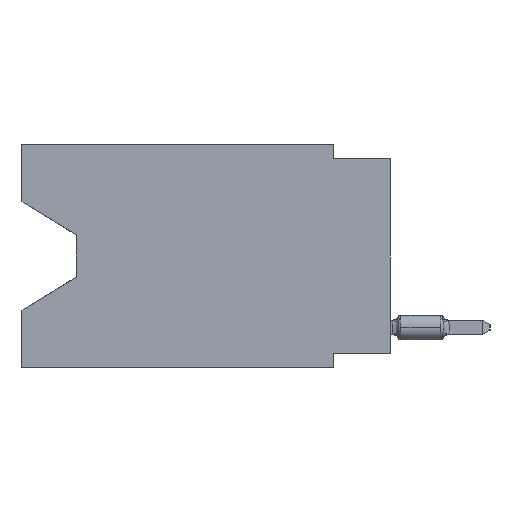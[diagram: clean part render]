
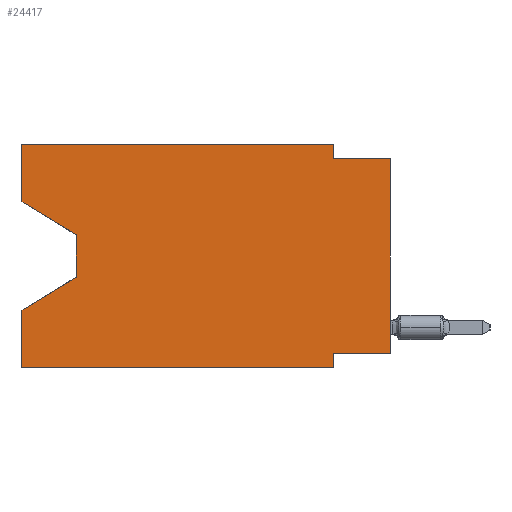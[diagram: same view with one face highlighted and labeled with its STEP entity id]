
A CAD part, left-side view. The second image highlights one B-rep face of the part: STEP entity #24417.
In plain terms, the highlighted planar face has unit normal (-1, 0, 0).
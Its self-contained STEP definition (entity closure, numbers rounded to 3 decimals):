
#320 = CARTESIAN_POINT ( 'NONE',  ( 0., 2.54, -9.906 ) ) ;
#419 = ORIENTED_EDGE ( 'NONE', *, *, #29567, .F. ) ;
#434 = VERTEX_POINT ( 'NONE', #31458 ) ;
#582 = CARTESIAN_POINT ( 'NONE',  ( 0., 16.383, -2.546 ) ) ;
#622 = LINE ( 'NONE', #24357, #13820 ) ;
#1254 = LINE ( 'NONE', #16887, #22067 ) ;
#1901 = ORIENTED_EDGE ( 'NONE', *, *, #32704, .F. ) ;
#2399 = DIRECTION ( 'NONE',  ( 0., 0., 1. ) ) ;
#2445 = ORIENTED_EDGE ( 'NONE', *, *, #22307, .F. ) ;
#2639 = VERTEX_POINT ( 'NONE', #28335 ) ;
#2742 = CARTESIAN_POINT ( 'NONE',  ( 0., 16.383, 0. ) ) ;
#2745 = ORIENTED_EDGE ( 'NONE', *, *, #31666, .T. ) ;
#2800 = VECTOR ( 'NONE', #32948, 1000. ) ;
#3052 = ORIENTED_EDGE ( 'NONE', *, *, #31285, .T. ) ;
#3186 = LINE ( 'NONE', #11596, #4100 ) ;
#3419 = EDGE_CURVE ( 'NONE', #2639, #34165, #1254, .T. ) ;
#3425 = EDGE_CURVE ( 'NONE', #27504, #32632, #14602, .T. ) ;
#4008 = ORIENTED_EDGE ( 'NONE', *, *, #20793, .F. ) ;
#4100 = VECTOR ( 'NONE', #17050, 1000. ) ;
#4119 = CARTESIAN_POINT ( 'NONE',  ( 0., 2.54, -9.271 ) ) ;
#5237 = VECTOR ( 'NONE', #19702, 1000. ) ;
#5678 = CARTESIAN_POINT ( 'NONE',  ( 0., 16.383, 0. ) ) ;
#5888 = VECTOR ( 'NONE', #28918, 1000. ) ;
#8313 = LINE ( 'NONE', #5678, #13576 ) ;
#8355 = CARTESIAN_POINT ( 'NONE',  ( 0., 16.383, -9.906 ) ) ;
#9902 = LINE ( 'NONE', #23429, #23069 ) ;
#10586 = ORIENTED_EDGE ( 'NONE', *, *, #19698, .F. ) ;
#10642 = CARTESIAN_POINT ( 'NONE',  ( 0., 2.54, 0. ) ) ;
#11029 = DIRECTION ( 'NONE',  ( 0., 0., -1. ) ) ;
#11428 = DIRECTION ( 'NONE',  ( 0., 0., 1. ) ) ;
#11596 = CARTESIAN_POINT ( 'NONE',  ( 0., 0., -0.635 ) ) ;
#12341 = CARTESIAN_POINT ( 'NONE',  ( 0., 16.383, -7.36 ) ) ;
#12742 = CARTESIAN_POINT ( 'NONE',  ( 0., 13.97, -5.893 ) ) ;
#12878 = DIRECTION ( 'NONE',  ( 0., 0., -1. ) ) ;
#13576 = VECTOR ( 'NONE', #27130, 1000. ) ;
#13820 = VECTOR ( 'NONE', #19258, 1000. ) ;
#13827 = VECTOR ( 'NONE', #11029, 1000. ) ;
#14162 = CARTESIAN_POINT ( 'NONE',  ( 0., 16.383, 0. ) ) ;
#14336 = LINE ( 'NONE', #21589, #2800 ) ;
#14414 = FACE_OUTER_BOUND ( 'NONE', #19501, .T. ) ;
#14585 = DIRECTION ( 'NONE',  ( 1., 0., 0. ) ) ;
#14602 = LINE ( 'NONE', #30751, #5237 ) ;
#16218 = VERTEX_POINT ( 'NONE', #21781 ) ;
#16665 = VERTEX_POINT ( 'NONE', #12341 ) ;
#16887 = CARTESIAN_POINT ( 'NONE',  ( 0., 0., 0. ) ) ;
#17050 = DIRECTION ( 'NONE',  ( 0., -1., 0. ) ) ;
#17220 = PLANE ( 'NONE',  #29820 ) ;
#17587 = DIRECTION ( 'NONE',  ( 0., -0.855, -0.519 ) ) ;
#17879 = VECTOR ( 'NONE', #27169, 1000. ) ;
#18353 = CARTESIAN_POINT ( 'NONE',  ( 0., 0., -0.635 ) ) ;
#19258 = DIRECTION ( 'NONE',  ( 0., -1., 0. ) ) ;
#19458 = VERTEX_POINT ( 'NONE', #28154 ) ;
#19501 = EDGE_LOOP ( 'NONE', ( #2745, #30561, #34324, #31745, #3052, #419, #1901, #31665, #10586, #2445, #21273, #4008 ) ) ;
#19682 = CARTESIAN_POINT ( 'NONE',  ( 0., 16.383, 0. ) ) ;
#19698 = EDGE_CURVE ( 'NONE', #26104, #34165, #3186, .T. ) ;
#19702 = DIRECTION ( 'NONE',  ( 0., -1., 0. ) ) ;
#20224 = LINE ( 'NONE', #23204, #25614 ) ;
#20793 = EDGE_CURVE ( 'NONE', #33190, #27504, #26462, .T. ) ;
#21034 = VERTEX_POINT ( 'NONE', #4119 ) ;
#21273 = ORIENTED_EDGE ( 'NONE', *, *, #3425, .F. ) ;
#21589 = CARTESIAN_POINT ( 'NONE',  ( 0., 13.97, -4.013 ) ) ;
#21781 = CARTESIAN_POINT ( 'NONE',  ( 0., 2.54, -9.906 ) ) ;
#22067 = VECTOR ( 'NONE', #11428, 1000. ) ;
#22307 = EDGE_CURVE ( 'NONE', #32632, #26104, #9902, .T. ) ;
#22469 = EDGE_CURVE ( 'NONE', #31222, #16665, #8313, .T. ) ;
#23069 = VECTOR ( 'NONE', #12878, 1000. ) ;
#23204 = CARTESIAN_POINT ( 'NONE',  ( 0., 16.383, -2.546 ) ) ;
#23429 = CARTESIAN_POINT ( 'NONE',  ( 0., 2.54, 0. ) ) ;
#23546 = VECTOR ( 'NONE', #2399, 1000. ) ;
#24357 = CARTESIAN_POINT ( 'NONE',  ( 0., 16.383, -9.906 ) ) ;
#24417 = ADVANCED_FACE ( 'NONE', ( #14414 ), #17220, .F. ) ;
#25614 = VECTOR ( 'NONE', #17587, 1000. ) ;
#26104 = VERTEX_POINT ( 'NONE', #28411 ) ;
#26462 = LINE ( 'NONE', #2742, #23546 ) ;
#26990 = LINE ( 'NONE', #29791, #17879 ) ;
#27130 = DIRECTION ( 'NONE',  ( 0., 0., 1. ) ) ;
#27169 = DIRECTION ( 'NONE',  ( 0., 1., 0. ) ) ;
#27377 = LINE ( 'NONE', #320, #13827 ) ;
#27504 = VERTEX_POINT ( 'NONE', #14162 ) ;
#28145 = EDGE_CURVE ( 'NONE', #434, #16665, #28230, .T. ) ;
#28154 = CARTESIAN_POINT ( 'NONE',  ( 0., 13.97, -4.013 ) ) ;
#28230 = LINE ( 'NONE', #12742, #5888 ) ;
#28335 = CARTESIAN_POINT ( 'NONE',  ( 0., 0., -9.271 ) ) ;
#28411 = CARTESIAN_POINT ( 'NONE',  ( 0., 2.54, -0.635 ) ) ;
#28918 = DIRECTION ( 'NONE',  ( 0., 0.855, -0.519 ) ) ;
#29567 = EDGE_CURVE ( 'NONE', #21034, #16218, #27377, .T. ) ;
#29791 = CARTESIAN_POINT ( 'NONE',  ( 0., 0., -9.271 ) ) ;
#29820 = AXIS2_PLACEMENT_3D ( 'NONE', #19682, #14585, #30736 ) ;
#30561 = ORIENTED_EDGE ( 'NONE', *, *, #33911, .T. ) ;
#30736 = DIRECTION ( 'NONE',  ( 0., 0., -1. ) ) ;
#30751 = CARTESIAN_POINT ( 'NONE',  ( 0., 16.383, 0. ) ) ;
#31222 = VERTEX_POINT ( 'NONE', #8355 ) ;
#31285 = EDGE_CURVE ( 'NONE', #31222, #16218, #622, .T. ) ;
#31458 = CARTESIAN_POINT ( 'NONE',  ( 0., 13.97, -5.893 ) ) ;
#31665 = ORIENTED_EDGE ( 'NONE', *, *, #3419, .T. ) ;
#31666 = EDGE_CURVE ( 'NONE', #33190, #19458, #20224, .T. ) ;
#31745 = ORIENTED_EDGE ( 'NONE', *, *, #22469, .F. ) ;
#32632 = VERTEX_POINT ( 'NONE', #10642 ) ;
#32704 = EDGE_CURVE ( 'NONE', #2639, #21034, #26990, .T. ) ;
#32948 = DIRECTION ( 'NONE',  ( 0., 0., -1. ) ) ;
#33190 = VERTEX_POINT ( 'NONE', #582 ) ;
#33911 = EDGE_CURVE ( 'NONE', #19458, #434, #14336, .T. ) ;
#34165 = VERTEX_POINT ( 'NONE', #18353 ) ;
#34324 = ORIENTED_EDGE ( 'NONE', *, *, #28145, .T. ) ;
